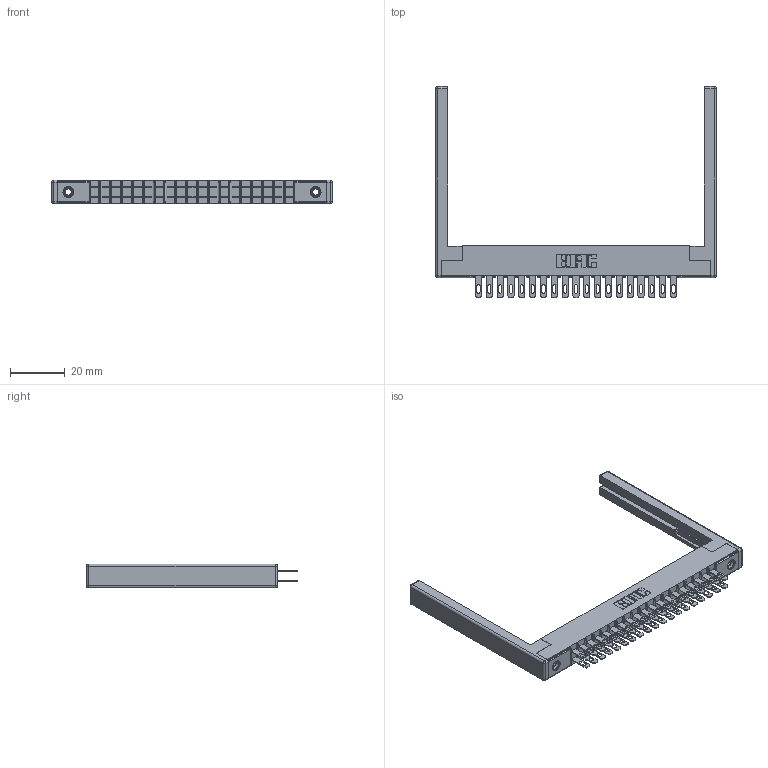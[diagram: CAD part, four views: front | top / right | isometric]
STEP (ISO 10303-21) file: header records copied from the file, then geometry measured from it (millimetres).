
FILE_DESCRIPTION (( 'STEP AP203' ), '1' );
FILE_NAME ('305-038-500-268.STEP', '2019-09-09T18:20:35', ( '' ), ( '' ), 'SwSTEP 2.0', 'SolidWorks 2016', '' );
FILE_SCHEMA (( 'CONFIG_CONTROL_DESIGN' ));
Length unit declared in the file: inch
Products named in the file (5): 345-250-001_345-250-001-102; 307-220-068; 305-038-500-268; 305-290-001_500; 305 Part_.156 Dia
Assembly tree (43 placements, depth 2):
  305-038-500-268
    305 Part_.156 Dia
    305-290-001_500  x38
    345-250-001_345-250-001-102  x2
    307-220-068  x2
Bounding box: 102.72 x 77.14 x 8.71 mm (x, y, z)
Volume: 11133.4 mm3; surface area: 16923.3 mm2
Topology: 43 solids, 43 shells, 2170 faces, 6159 edges, 3982 vertices
Faces by surface type: plane 1220, cylinder 850, sphere 84, cone 12, torus 4
Entity records: 26153 total; most frequent: CARTESIAN_POINT 4300, ORIENTED_EDGE 4256, DIRECTION 4200, EDGE_CURVE 2128, LINE 1684, VECTOR 1684, VERTEX_POINT 1358, AXIS2_PLACEMENT_3D 1258
